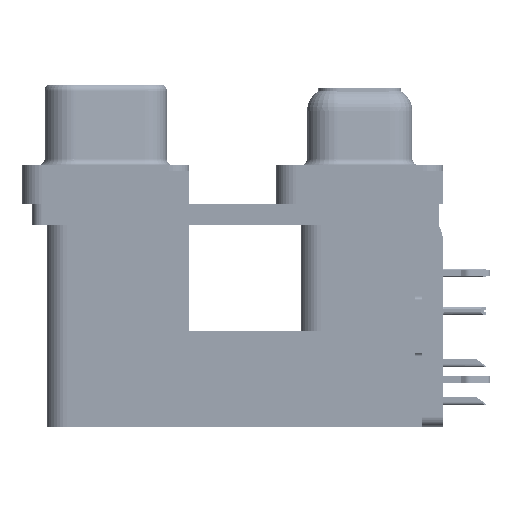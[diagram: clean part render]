
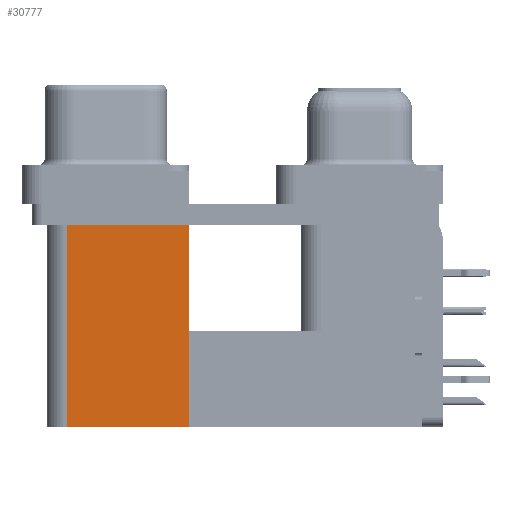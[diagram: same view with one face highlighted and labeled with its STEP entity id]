
A CAD part, left-side view. The second image highlights one B-rep face of the part: STEP entity #30777.
In plain terms, the highlighted planar face has unit normal (-1, 0, 0).
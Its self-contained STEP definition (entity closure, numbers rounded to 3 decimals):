
#3755 = DIRECTION ( 'NONE',  ( 0., 1., 0. ) ) ;
#4326 = CARTESIAN_POINT ( 'NONE',  ( 3.79, 12.775, -19.2 ) ) ;
#9496 = EDGE_LOOP ( 'NONE', ( #22248, #28223, #43310, #32888 ) ) ;
#12610 = AXIS2_PLACEMENT_3D ( 'NONE', #24080, #49791, #3755 ) ;
#13309 = LINE ( 'NONE', #48679, #48914 ) ;
#13702 = VECTOR ( 'NONE', #39921, 1000. ) ;
#17810 = DIRECTION ( 'NONE',  ( 0., 1., 0. ) ) ;
#18591 = FACE_OUTER_BOUND ( 'NONE', #9496, .T. ) ;
#19053 = CARTESIAN_POINT ( 'NONE',  ( 3.79, 12.775, -19.2 ) ) ;
#19891 = VERTEX_POINT ( 'NONE', #39615 ) ;
#22248 = ORIENTED_EDGE ( 'NONE', *, *, #45747, .T. ) ;
#23098 = CARTESIAN_POINT ( 'NONE',  ( 3.79, 12.775, -2.5 ) ) ;
#24080 = CARTESIAN_POINT ( 'NONE',  ( 3.79, 12.775, -19.2 ) ) ;
#24496 = LINE ( 'NONE', #65995, #13702 ) ;
#28223 = ORIENTED_EDGE ( 'NONE', *, *, #30382, .F. ) ;
#30382 = EDGE_CURVE ( 'NONE', #47342, #19891, #24496, .T. ) ;
#30777 = ADVANCED_FACE ( 'NONE', ( #18591 ), #44993, .F. ) ;
#32888 = ORIENTED_EDGE ( 'NONE', *, *, #41534, .T. ) ;
#33701 = VERTEX_POINT ( 'NONE', #23098 ) ;
#35461 = LINE ( 'NONE', #36142, #58011 ) ;
#36142 = CARTESIAN_POINT ( 'NONE',  ( 3.79, 12.775, -19.2 ) ) ;
#39615 = CARTESIAN_POINT ( 'NONE',  ( 3.79, 21.975, -2.5 ) ) ;
#39623 = LINE ( 'NONE', #19053, #62931 ) ;
#39921 = DIRECTION ( 'NONE',  ( 0., 0., 1. ) ) ;
#41534 = EDGE_CURVE ( 'NONE', #42408, #33701, #39623, .T. ) ;
#42408 = VERTEX_POINT ( 'NONE', #4326 ) ;
#43310 = ORIENTED_EDGE ( 'NONE', *, *, #49363, .F. ) ;
#44993 = PLANE ( 'NONE',  #12610 ) ;
#45747 = EDGE_CURVE ( 'NONE', #33701, #19891, #13309, .T. ) ;
#47342 = VERTEX_POINT ( 'NONE', #48614 ) ;
#48614 = CARTESIAN_POINT ( 'NONE',  ( 3.79, 21.975, -19.2 ) ) ;
#48679 = CARTESIAN_POINT ( 'NONE',  ( 3.79, 12.775, -2.5 ) ) ;
#48914 = VECTOR ( 'NONE', #17810, 1000. ) ;
#49363 = EDGE_CURVE ( 'NONE', #42408, #47342, #35461, .T. ) ;
#49577 = DIRECTION ( 'NONE',  ( 0., 0., 1. ) ) ;
#49791 = DIRECTION ( 'NONE',  ( 1., 0., 0. ) ) ;
#52263 = DIRECTION ( 'NONE',  ( 0., 1., 0. ) ) ;
#58011 = VECTOR ( 'NONE', #52263, 1000. ) ;
#62931 = VECTOR ( 'NONE', #49577, 1000. ) ;
#65995 = CARTESIAN_POINT ( 'NONE',  ( 3.79, 21.975, -19.2 ) ) ;
